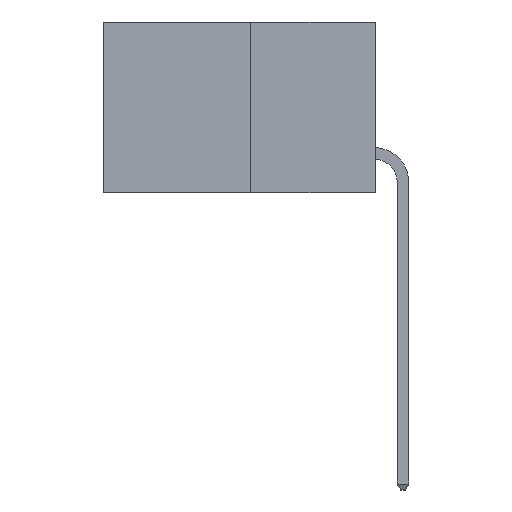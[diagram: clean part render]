
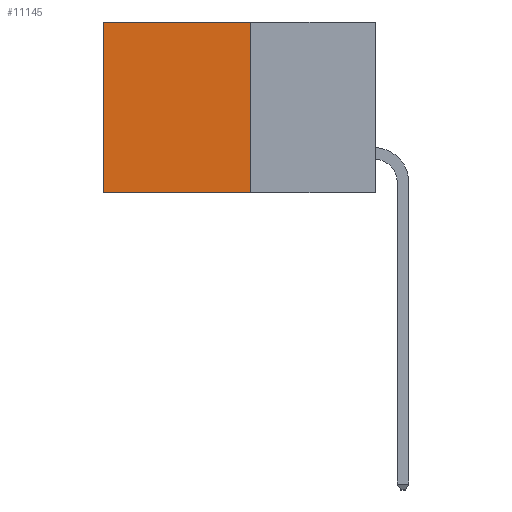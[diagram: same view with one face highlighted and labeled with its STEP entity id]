
A CAD part, left-side view. The second image highlights one B-rep face of the part: STEP entity #11145.
In plain terms, the highlighted planar face has unit normal (-1, 0, 0).
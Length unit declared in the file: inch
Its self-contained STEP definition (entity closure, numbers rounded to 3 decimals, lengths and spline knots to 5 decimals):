
#922 = ORIENTED_EDGE ( 'NONE', *, *, #2125, .F. ) ;
#1146 = CARTESIAN_POINT ( 'NONE',  ( 0.277, 0.27, -0.37 ) ) ;
#1229 = CARTESIAN_POINT ( 'NONE',  ( 0.277, 0.59, -0.37 ) ) ;
#1319 = VECTOR ( 'NONE', #2391, 39.37008 ) ;
#1347 = ORIENTED_EDGE ( 'NONE', *, *, #8811, .F. ) ;
#1409 = DIRECTION ( 'NONE',  ( 0., 1., 0. ) ) ;
#1660 = CARTESIAN_POINT ( 'NONE',  ( 0.277, 0.27, -0.37 ) ) ;
#1766 = AXIS2_PLACEMENT_3D ( 'NONE', #1660, #2589, #9173 ) ;
#2038 = ORIENTED_EDGE ( 'NONE', *, *, #6562, .T. ) ;
#2125 = EDGE_CURVE ( 'NONE', #3971, #8118, #10334, .T. ) ;
#2391 = DIRECTION ( 'NONE',  ( 0., 0., -1. ) ) ;
#2589 = DIRECTION ( 'NONE',  ( 1., 0., 0. ) ) ;
#2740 = VECTOR ( 'NONE', #11530, 39.37008 ) ;
#2825 = VECTOR ( 'NONE', #1409, 39.37008 ) ;
#3944 = FACE_OUTER_BOUND ( 'NONE', #10308, .T. ) ;
#3971 = VERTEX_POINT ( 'NONE', #9626 ) ;
#4269 = ORIENTED_EDGE ( 'NONE', *, *, #5226, .T. ) ;
#4580 = VERTEX_POINT ( 'NONE', #9150 ) ;
#5226 = EDGE_CURVE ( 'NONE', #6302, #4580, #7762, .T. ) ;
#6048 = LINE ( 'NONE', #7116, #1319 ) ;
#6302 = VERTEX_POINT ( 'NONE', #9370 ) ;
#6562 = EDGE_CURVE ( 'NONE', #4580, #8118, #9805, .T. ) ;
#7116 = CARTESIAN_POINT ( 'NONE',  ( 0.277, 0.27, -0.37 ) ) ;
#7308 = PLANE ( 'NONE',  #1766 ) ;
#7313 = VECTOR ( 'NONE', #7707, 39.37008 ) ;
#7707 = DIRECTION ( 'NONE',  ( 0., 0., -1. ) ) ;
#7762 = LINE ( 'NONE', #11516, #2740 ) ;
#7797 = CARTESIAN_POINT ( 'NONE',  ( 0.277, 0.59, -0.37 ) ) ;
#8118 = VERTEX_POINT ( 'NONE', #1229 ) ;
#8811 = EDGE_CURVE ( 'NONE', #6302, #3971, #6048, .T. ) ;
#9150 = CARTESIAN_POINT ( 'NONE',  ( 0.277, 0.59, 0. ) ) ;
#9173 = DIRECTION ( 'NONE',  ( 0., 0., -1. ) ) ;
#9370 = CARTESIAN_POINT ( 'NONE',  ( 0.277, 0.27, 0. ) ) ;
#9626 = CARTESIAN_POINT ( 'NONE',  ( 0.277, 0.27, -0.37 ) ) ;
#9805 = LINE ( 'NONE', #7797, #7313 ) ;
#10308 = EDGE_LOOP ( 'NONE', ( #2038, #922, #1347, #4269 ) ) ;
#10334 = LINE ( 'NONE', #1146, #2825 ) ;
#11145 = ADVANCED_FACE ( 'NONE', ( #3944 ), #7308, .F. ) ;
#11516 = CARTESIAN_POINT ( 'NONE',  ( 0.277, 0.27, 0. ) ) ;
#11530 = DIRECTION ( 'NONE',  ( 0., 1., 0. ) ) ;
